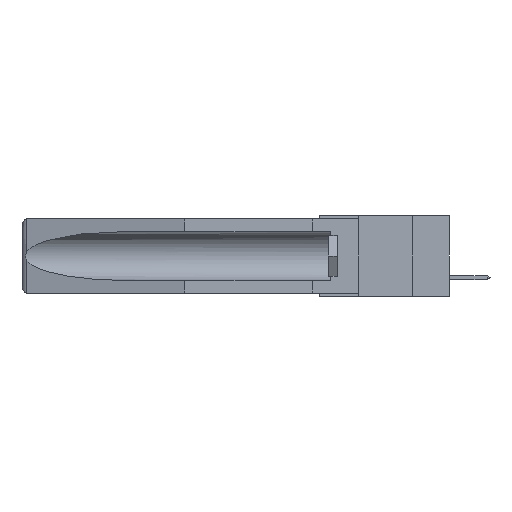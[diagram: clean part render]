
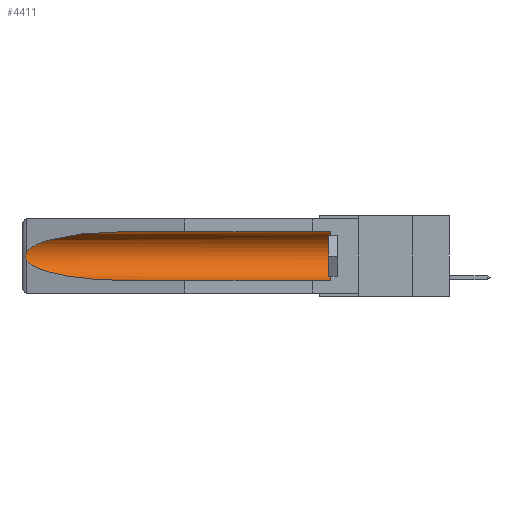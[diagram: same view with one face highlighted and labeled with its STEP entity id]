
A CAD part, left-side view. The second image highlights one B-rep face of the part: STEP entity #4411.
In plain terms, the highlighted cylindrical face has radius 2.857 mm (diameter 5.715 mm), a partial arc.
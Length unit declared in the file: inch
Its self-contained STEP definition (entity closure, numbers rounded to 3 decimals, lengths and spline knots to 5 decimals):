
#644 =( BOUNDED_CURVE ( )  B_SPLINE_CURVE ( 3, ( #20306, #26917, #16610, #3122 ),
 .UNSPECIFIED., .F., .F. ) 
 B_SPLINE_CURVE_WITH_KNOTS ( ( 4, 4 ),
 ( 0.1948, 1.5708 ),
 .UNSPECIFIED. ) 
 CURVE ( )  GEOMETRIC_REPRESENTATION_ITEM ( )  RATIONAL_B_SPLINE_CURVE ( ( 1., 0.848, 0.848, 1. ) ) 
 REPRESENTATION_ITEM ( '' )  );
#897 = CARTESIAN_POINT ( 'NONE',  ( 0.2675, 1.53308, -0.17534 ) ) ;
#1430 = ORIENTED_EDGE ( 'NONE', *, *, #9430, .T. ) ;
#3095 = CARTESIAN_POINT ( 'NONE',  ( 0.2673, 1.53269, -0.17917 ) ) ;
#3122 = CARTESIAN_POINT ( 'NONE',  ( 0.155, 1.07973, -0.284 ) ) ;
#3202 = CARTESIAN_POINT ( 'NONE',  ( 0.26597, 1.5296, -0.19026 ) ) ;
#3206 = DIRECTION ( 'NONE',  ( 0., 1., 0. ) ) ;
#3629 = B_SPLINE_CURVE_WITH_KNOTS ( 'NONE', 3,
 ( #11644, #9549, #13875, #11941, #11742, #897, #3095, #16380, #3202, #20752 ),
 .UNSPECIFIED., .F., .F.,
 ( 4, 2, 2, 2, 4 ),
 ( 0., 0.00029, 0.00058, 0.00087, 0.00117 ),
 .UNSPECIFIED. ) ;
#4043 = AXIS2_PLACEMENT_3D ( 'NONE', #4444, #17540, #6346 ) ;
#4113 = CARTESIAN_POINT ( 'NONE',  ( 0.155, -0.30754, -0.059 ) ) ;
#4176 = CARTESIAN_POINT ( 'NONE',  ( 0.155, 0.126, -0.284 ) ) ;
#4411 = ADVANCED_FACE ( 'NONE', ( #18685 ), #22118, .F. ) ;
#4444 = CARTESIAN_POINT ( 'NONE',  ( 0.155, 0.126, -0.1715 ) ) ;
#5073 = LINE ( 'NONE', #19825, #7842 ) ;
#6346 = DIRECTION ( 'NONE',  ( 0., 0., 1. ) ) ;
#6422 = ORIENTED_EDGE ( 'NONE', *, *, #20049, .T. ) ;
#6797 = CARTESIAN_POINT ( 'NONE',  ( 0.26537, 1.52718, -0.14972 ) ) ;
#7167 = EDGE_CURVE ( 'NONE', #23537, #10347, #3629, .T. ) ;
#7842 = VECTOR ( 'NONE', #14458, 39.37008 ) ;
#8183 = CARTESIAN_POINT ( 'NONE',  ( 0.25451, 1.48313, -0.09465 ) ) ;
#8548 = VERTEX_POINT ( 'NONE', #23365 ) ;
#8771 = AXIS2_PLACEMENT_3D ( 'NONE', #20855, #3206, #27357 ) ;
#9430 = EDGE_CURVE ( 'NONE', #17616, #8548, #26470, .T. ) ;
#9549 = CARTESIAN_POINT ( 'NONE',  ( 0.26597, 1.52961, -0.15275 ) ) ;
#10347 = VERTEX_POINT ( 'NONE', #24196 ) ;
#11644 = CARTESIAN_POINT ( 'NONE',  ( 0.26537, 1.52718, -0.14972 ) ) ;
#11742 = CARTESIAN_POINT ( 'NONE',  ( 0.2675, 1.53308, -0.16763 ) ) ;
#11941 = CARTESIAN_POINT ( 'NONE',  ( 0.2673, 1.5327, -0.16383 ) ) ;
#12772 = EDGE_CURVE ( 'NONE', #21708, #24986, #5073, .T. ) ;
#12867 = ORIENTED_EDGE ( 'NONE', *, *, #24249, .T. ) ;
#13853 =( BOUNDED_CURVE ( )  B_SPLINE_CURVE ( 3, ( #19226, #21123, #8183, #23532 ),
 .UNSPECIFIED., .F., .F. ) 
 B_SPLINE_CURVE_WITH_KNOTS ( ( 4, 4 ),
 ( 4.71239, 6.08839 ),
 .UNSPECIFIED. ) 
 CURVE ( )  GEOMETRIC_REPRESENTATION_ITEM ( )  RATIONAL_B_SPLINE_CURVE ( ( 1., 0.848, 0.848, 1. ) ) 
 REPRESENTATION_ITEM ( '' )  );
#13875 = CARTESIAN_POINT ( 'NONE',  ( 0.26654, 1.53092, -0.15636 ) ) ;
#14458 = DIRECTION ( 'NONE',  ( 0., 1., 0. ) ) ;
#14835 = CARTESIAN_POINT ( 'NONE',  ( 0.155, 1.07973, -0.284 ) ) ;
#16197 = ORIENTED_EDGE ( 'NONE', *, *, #17051, .T. ) ;
#16380 = CARTESIAN_POINT ( 'NONE',  ( 0.26655, 1.53094, -0.18657 ) ) ;
#16610 = CARTESIAN_POINT ( 'NONE',  ( 0.21114, 1.30732, -0.284 ) ) ;
#17051 = EDGE_CURVE ( 'NONE', #10347, #24986, #644, .T. ) ;
#17540 = DIRECTION ( 'NONE',  ( 0., -1., 0. ) ) ;
#17616 = VERTEX_POINT ( 'NONE', #24169 ) ;
#18430 = ORIENTED_EDGE ( 'NONE', *, *, #12772, .F. ) ;
#18685 = FACE_OUTER_BOUND ( 'NONE', #19039, .T. ) ;
#18921 = VECTOR ( 'NONE', #19102, 39.37008 ) ;
#19039 = EDGE_LOOP ( 'NONE', ( #12867, #23400, #16197, #18430, #6422, #1430 ) ) ;
#19102 = DIRECTION ( 'NONE',  ( 0., 1., 0. ) ) ;
#19226 = CARTESIAN_POINT ( 'NONE',  ( 0.155, 1.07973, -0.059 ) ) ;
#19825 = CARTESIAN_POINT ( 'NONE',  ( 0.155, -0.30754, -0.284 ) ) ;
#20049 = EDGE_CURVE ( 'NONE', #21708, #17616, #26519, .T. ) ;
#20306 = CARTESIAN_POINT ( 'NONE',  ( 0.26537, 1.52718, -0.19328 ) ) ;
#20752 = CARTESIAN_POINT ( 'NONE',  ( 0.26537, 1.52718, -0.19328 ) ) ;
#20855 = CARTESIAN_POINT ( 'NONE',  ( 0.155, -0.30754, -0.1715 ) ) ;
#21123 = CARTESIAN_POINT ( 'NONE',  ( 0.21114, 1.30732, -0.059 ) ) ;
#21708 = VERTEX_POINT ( 'NONE', #4176 ) ;
#22118 = CYLINDRICAL_SURFACE ( 'NONE', #8771, 0.1125 ) ;
#23365 = CARTESIAN_POINT ( 'NONE',  ( 0.155, 1.07973, -0.059 ) ) ;
#23400 = ORIENTED_EDGE ( 'NONE', *, *, #7167, .T. ) ;
#23532 = CARTESIAN_POINT ( 'NONE',  ( 0.26537, 1.52718, -0.14972 ) ) ;
#23537 = VERTEX_POINT ( 'NONE', #6797 ) ;
#24169 = CARTESIAN_POINT ( 'NONE',  ( 0.155, 0.126, -0.059 ) ) ;
#24196 = CARTESIAN_POINT ( 'NONE',  ( 0.26537, 1.52718, -0.19328 ) ) ;
#24249 = EDGE_CURVE ( 'NONE', #8548, #23537, #13853, .T. ) ;
#24986 = VERTEX_POINT ( 'NONE', #14835 ) ;
#26470 = LINE ( 'NONE', #4113, #18921 ) ;
#26519 = CIRCLE ( 'NONE', #4043, 0.1125 ) ;
#26917 = CARTESIAN_POINT ( 'NONE',  ( 0.25451, 1.48313, -0.24835 ) ) ;
#27357 = DIRECTION ( 'NONE',  ( 0., 0., 1. ) ) ;
